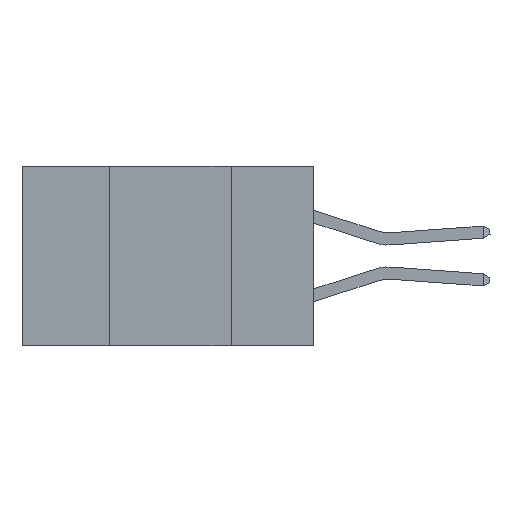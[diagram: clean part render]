
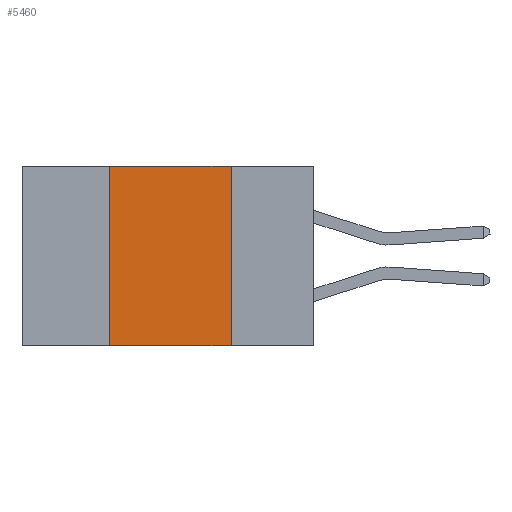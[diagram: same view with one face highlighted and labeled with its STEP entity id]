
A CAD part, left-side view. The second image highlights one B-rep face of the part: STEP entity #5460.
In plain terms, the highlighted planar face has unit normal (-1, 0, 0).
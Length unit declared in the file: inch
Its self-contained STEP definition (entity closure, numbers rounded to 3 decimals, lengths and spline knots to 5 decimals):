
#1822 = VERTEX_POINT ( 'NONE', #3851 ) ;
#2988 = FACE_OUTER_BOUND ( 'NONE', #6671, .T. ) ;
#3851 = CARTESIAN_POINT ( 'NONE',  ( 0., 0.42, 0. ) ) ;
#5460 = ADVANCED_FACE ( 'NONE', ( #2988 ), #6455, .F. ) ;
#6228 = LINE ( 'NONE', #16830, #8528 ) ;
#6455 = PLANE ( 'NONE',  #34332 ) ;
#6671 = EDGE_LOOP ( 'NONE', ( #17304, #28941, #31416, #21656 ) ) ;
#6791 = CARTESIAN_POINT ( 'NONE',  ( 0., 0.6, 0. ) ) ;
#8528 = VECTOR ( 'NONE', #33500, 39.37008 ) ;
#9274 = DIRECTION ( 'NONE',  ( 1., 0., 0. ) ) ;
#10349 = EDGE_CURVE ( 'NONE', #34967, #36726, #32857, .T. ) ;
#11446 = EDGE_CURVE ( 'NONE', #1822, #21902, #36645, .T. ) ;
#16410 = CARTESIAN_POINT ( 'NONE',  ( 0., 0.6, -0.37 ) ) ;
#16736 = DIRECTION ( 'NONE',  ( 0., -1., 0. ) ) ;
#16830 = CARTESIAN_POINT ( 'NONE',  ( 0., 0.42, 0. ) ) ;
#17304 = ORIENTED_EDGE ( 'NONE', *, *, #39634, .F. ) ;
#18161 = CARTESIAN_POINT ( 'NONE',  ( 0., 0.42, -0.37 ) ) ;
#19213 = CARTESIAN_POINT ( 'NONE',  ( 0., 0.6, 0. ) ) ;
#19651 = DIRECTION ( 'NONE',  ( 0., 0., -1. ) ) ;
#21656 = ORIENTED_EDGE ( 'NONE', *, *, #10349, .T. ) ;
#21902 = VERTEX_POINT ( 'NONE', #32842 ) ;
#22683 = VECTOR ( 'NONE', #32728, 39.37008 ) ;
#26527 = EDGE_CURVE ( 'NONE', #34967, #1822, #6228, .T. ) ;
#26786 = CARTESIAN_POINT ( 'NONE',  ( 0., 0.17, -0.37 ) ) ;
#28941 = ORIENTED_EDGE ( 'NONE', *, *, #11446, .F. ) ;
#29897 = LINE ( 'NONE', #39629, #22683 ) ;
#31416 = ORIENTED_EDGE ( 'NONE', *, *, #26527, .F. ) ;
#32728 = DIRECTION ( 'NONE',  ( 0., 0., -1. ) ) ;
#32842 = CARTESIAN_POINT ( 'NONE',  ( 0., 0.17, 0. ) ) ;
#32857 = LINE ( 'NONE', #16410, #37887 ) ;
#33500 = DIRECTION ( 'NONE',  ( 0., 0., 1. ) ) ;
#33802 = VECTOR ( 'NONE', #16736, 39.37008 ) ;
#34332 = AXIS2_PLACEMENT_3D ( 'NONE', #19213, #9274, #19651 ) ;
#34967 = VERTEX_POINT ( 'NONE', #18161 ) ;
#36645 = LINE ( 'NONE', #6791, #33802 ) ;
#36726 = VERTEX_POINT ( 'NONE', #26786 ) ;
#37887 = VECTOR ( 'NONE', #38120, 39.37008 ) ;
#38120 = DIRECTION ( 'NONE',  ( 0., -1., 0. ) ) ;
#39629 = CARTESIAN_POINT ( 'NONE',  ( 0., 0.17, 0. ) ) ;
#39634 = EDGE_CURVE ( 'NONE', #21902, #36726, #29897, .T. ) ;
